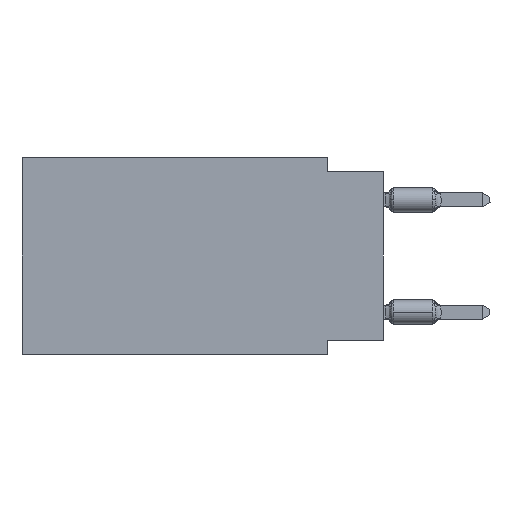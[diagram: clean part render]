
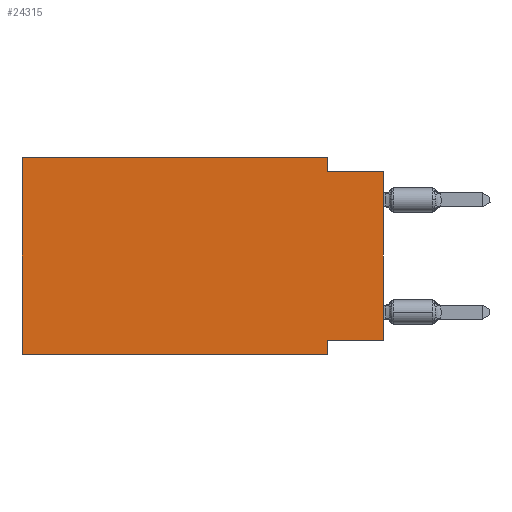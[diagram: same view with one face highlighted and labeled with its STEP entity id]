
A CAD part, left-side view. The second image highlights one B-rep face of the part: STEP entity #24315.
In plain terms, the highlighted planar face has unit normal (-1, 0, 0).
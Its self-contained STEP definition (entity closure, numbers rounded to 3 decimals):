
#299 = CARTESIAN_POINT ( 'NONE',  ( 0., 0., -8.255 ) ) ;
#462 = DIRECTION ( 'NONE',  ( 0., 1., 0. ) ) ;
#1142 = ORIENTED_EDGE ( 'NONE', *, *, #9440, .F. ) ;
#2275 = ORIENTED_EDGE ( 'NONE', *, *, #15096, .F. ) ;
#2407 = LINE ( 'NONE', #12961, #16599 ) ;
#2477 = EDGE_CURVE ( 'NONE', #8678, #6572, #10972, .T. ) ;
#2824 = LINE ( 'NONE', #21143, #24558 ) ;
#3416 = DIRECTION ( 'NONE',  ( 0., 0., -1. ) ) ;
#3806 = VERTEX_POINT ( 'NONE', #18304 ) ;
#4255 = LINE ( 'NONE', #17411, #14147 ) ;
#5271 = DIRECTION ( 'NONE',  ( 0., -1., 0. ) ) ;
#5300 = VECTOR ( 'NONE', #5271, 1000. ) ;
#6022 = DIRECTION ( 'NONE',  ( 1., 0., 0. ) ) ;
#6572 = VERTEX_POINT ( 'NONE', #6741 ) ;
#6741 = CARTESIAN_POINT ( 'NONE',  ( 0., 2.54, -8.89 ) ) ;
#7118 = EDGE_CURVE ( 'NONE', #8678, #27011, #25543, .T. ) ;
#7151 = CARTESIAN_POINT ( 'NONE',  ( 0., 2.54, -8.255 ) ) ;
#7848 = CARTESIAN_POINT ( 'NONE',  ( 0., 16.383, -8.89 ) ) ;
#8625 = CARTESIAN_POINT ( 'NONE',  ( 0., 16.383, 0. ) ) ;
#8678 = VERTEX_POINT ( 'NONE', #12858 ) ;
#8801 = EDGE_CURVE ( 'NONE', #29191, #6572, #2824, .T. ) ;
#9235 = ORIENTED_EDGE ( 'NONE', *, *, #31447, .T. ) ;
#9440 = EDGE_CURVE ( 'NONE', #25987, #10625, #12100, .T. ) ;
#9750 = EDGE_LOOP ( 'NONE', ( #9235, #1142, #2275, #18245, #13207, #11248, #23865, #27273 ) ) ;
#10625 = VERTEX_POINT ( 'NONE', #21264 ) ;
#10972 = LINE ( 'NONE', #7848, #5300 ) ;
#11248 = ORIENTED_EDGE ( 'NONE', *, *, #2477, .T. ) ;
#12067 = FACE_OUTER_BOUND ( 'NONE', #9750, .T. ) ;
#12100 = LINE ( 'NONE', #31092, #24530 ) ;
#12315 = VECTOR ( 'NONE', #23629, 1000. ) ;
#12858 = CARTESIAN_POINT ( 'NONE',  ( 0., 16.383, -8.89 ) ) ;
#12961 = CARTESIAN_POINT ( 'NONE',  ( 0., 0., 0. ) ) ;
#13207 = ORIENTED_EDGE ( 'NONE', *, *, #7118, .F. ) ;
#13444 = LINE ( 'NONE', #299, #15258 ) ;
#14147 = VECTOR ( 'NONE', #25525, 1000. ) ;
#14797 = AXIS2_PLACEMENT_3D ( 'NONE', #8625, #6022, #3416 ) ;
#15011 = VECTOR ( 'NONE', #16952, 1000. ) ;
#15096 = EDGE_CURVE ( 'NONE', #22182, #25987, #30084, .T. ) ;
#15258 = VECTOR ( 'NONE', #462, 1000. ) ;
#16144 = DIRECTION ( 'NONE',  ( 0., 0., -1. ) ) ;
#16599 = VECTOR ( 'NONE', #24723, 1000. ) ;
#16952 = DIRECTION ( 'NONE',  ( 0., 0., -1. ) ) ;
#17328 = EDGE_CURVE ( 'NONE', #3806, #29191, #13444, .T. ) ;
#17411 = CARTESIAN_POINT ( 'NONE',  ( 0., 16.383, 0. ) ) ;
#18245 = ORIENTED_EDGE ( 'NONE', *, *, #26087, .F. ) ;
#18304 = CARTESIAN_POINT ( 'NONE',  ( 0., 0., -8.255 ) ) ;
#19129 = CARTESIAN_POINT ( 'NONE',  ( 0., 2.54, -0.635 ) ) ;
#21143 = CARTESIAN_POINT ( 'NONE',  ( 0., 2.54, -8.89 ) ) ;
#21264 = CARTESIAN_POINT ( 'NONE',  ( 0., 0., -0.635 ) ) ;
#22182 = VERTEX_POINT ( 'NONE', #26238 ) ;
#22290 = CARTESIAN_POINT ( 'NONE',  ( 0., 2.54, 0. ) ) ;
#23629 = DIRECTION ( 'NONE',  ( 0., 0., 1. ) ) ;
#23865 = ORIENTED_EDGE ( 'NONE', *, *, #8801, .F. ) ;
#24315 = ADVANCED_FACE ( 'NONE', ( #12067 ), #32302, .F. ) ;
#24530 = VECTOR ( 'NONE', #30768, 1000. ) ;
#24558 = VECTOR ( 'NONE', #16144, 1000. ) ;
#24723 = DIRECTION ( 'NONE',  ( 0., 0., 1. ) ) ;
#25525 = DIRECTION ( 'NONE',  ( 0., -1., 0. ) ) ;
#25543 = LINE ( 'NONE', #25714, #12315 ) ;
#25714 = CARTESIAN_POINT ( 'NONE',  ( 0., 16.383, 0. ) ) ;
#25987 = VERTEX_POINT ( 'NONE', #19129 ) ;
#26087 = EDGE_CURVE ( 'NONE', #27011, #22182, #4255, .T. ) ;
#26238 = CARTESIAN_POINT ( 'NONE',  ( 0., 2.54, 0. ) ) ;
#27011 = VERTEX_POINT ( 'NONE', #28507 ) ;
#27273 = ORIENTED_EDGE ( 'NONE', *, *, #17328, .F. ) ;
#28507 = CARTESIAN_POINT ( 'NONE',  ( 0., 16.383, 0. ) ) ;
#29191 = VERTEX_POINT ( 'NONE', #7151 ) ;
#30084 = LINE ( 'NONE', #22290, #15011 ) ;
#30768 = DIRECTION ( 'NONE',  ( 0., -1., 0. ) ) ;
#31092 = CARTESIAN_POINT ( 'NONE',  ( 0., 0., -0.635 ) ) ;
#31447 = EDGE_CURVE ( 'NONE', #3806, #10625, #2407, .T. ) ;
#32302 = PLANE ( 'NONE',  #14797 ) ;
